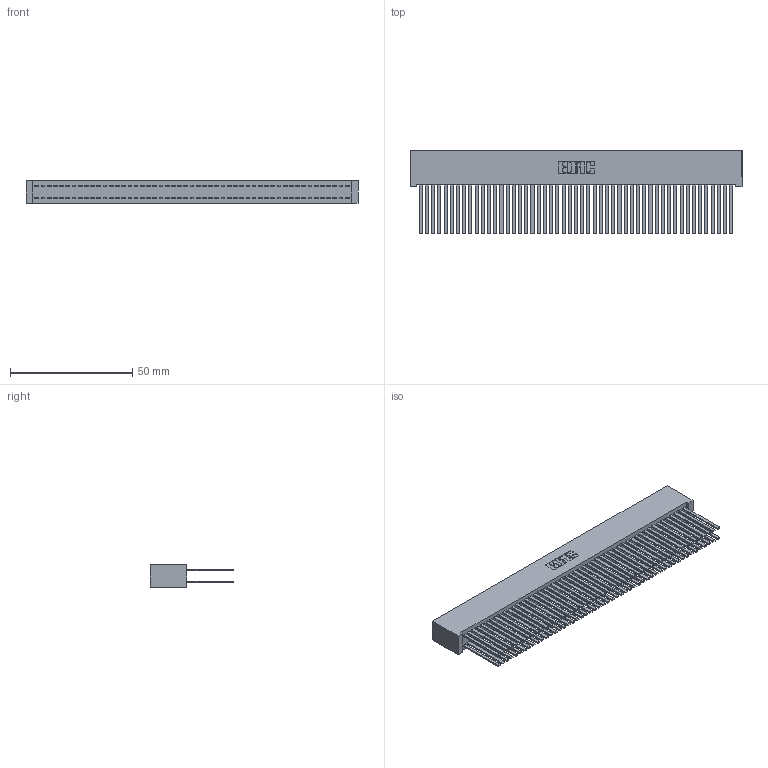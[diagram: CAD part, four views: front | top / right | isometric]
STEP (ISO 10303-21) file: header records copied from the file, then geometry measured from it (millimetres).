
FILE_DESCRIPTION (( 'STEP AP203' ), '1' );
FILE_NAME ('392-102-544-201.STEP', '2018-08-18T19:02:00', ( '' ), ( '' ), 'SwSTEP 2.0', 'SolidWorks 2016', '' );
FILE_SCHEMA (( 'CONFIG_CONTROL_DESIGN' ));
Length unit declared in the file: inch
Products named in the file (3): 342 Part_Lugless; 345-292-001_345-293-144; 392-102-544-201
Assembly tree (103 placements, depth 2):
  392-102-544-201
    342 Part_Lugless
    345-292-001_345-293-144  x102
Bounding box: 135.79 x 34.3 x 9.4 mm (x, y, z)
Volume: 14112.5 mm3; surface area: 27599.4 mm2
Topology: 103 solids, 103 shells, 4794 faces, 14249 edges, 9362 vertices
Faces by surface type: plane 3326, cylinder 1468
Entity records: 31053 total; most frequent: CARTESIAN_POINT 5130, ORIENTED_EDGE 5066, DIRECTION 4357, EDGE_CURVE 2533, VECTOR 2417, LINE 2417, VERTEX_POINT 1686, AXIS2_PLACEMENT_3D 970
